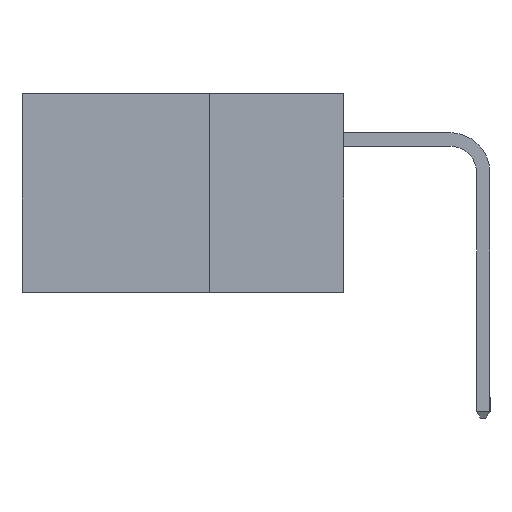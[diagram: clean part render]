
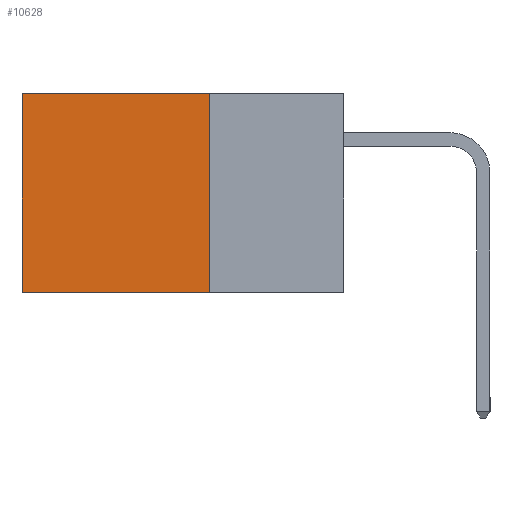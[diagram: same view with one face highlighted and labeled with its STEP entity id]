
A CAD part, left-side view. The second image highlights one B-rep face of the part: STEP entity #10628.
In plain terms, the highlighted planar face has unit normal (-1, 0, 0).
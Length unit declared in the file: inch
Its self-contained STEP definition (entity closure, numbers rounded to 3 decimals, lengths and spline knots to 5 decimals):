
#128 = CARTESIAN_POINT ( 'NONE',  ( 0.2615, 0.6, 0. ) ) ;
#481 = DIRECTION ( 'NONE',  ( 1., 0., 0. ) ) ;
#501 = LINE ( 'NONE', #14628, #19269 ) ;
#578 = EDGE_CURVE ( 'NONE', #7207, #7110, #7001, .T. ) ;
#1462 = CARTESIAN_POINT ( 'NONE',  ( 0.2615, 0.25, -0.37 ) ) ;
#2629 = VECTOR ( 'NONE', #13078, 39.37008 ) ;
#3656 = CARTESIAN_POINT ( 'NONE',  ( 0.2615, 0.6, -0.37 ) ) ;
#3917 = AXIS2_PLACEMENT_3D ( 'NONE', #11691, #481, #13597 ) ;
#5743 = EDGE_CURVE ( 'NONE', #24063, #7207, #501, .T. ) ;
#6727 = LINE ( 'NONE', #1462, #16217 ) ;
#7001 = LINE ( 'NONE', #16262, #2629 ) ;
#7110 = VERTEX_POINT ( 'NONE', #3656 ) ;
#7207 = VERTEX_POINT ( 'NONE', #128 ) ;
#8527 = ORIENTED_EDGE ( 'NONE', *, *, #578, .T. ) ;
#10224 = DIRECTION ( 'NONE',  ( 0., 1., 0. ) ) ;
#10291 = ORIENTED_EDGE ( 'NONE', *, *, #17161, .F. ) ;
#10628 = ADVANCED_FACE ( 'NONE', ( #15994 ), #22792, .F. ) ;
#10825 = CARTESIAN_POINT ( 'NONE',  ( 0.2615, 0.25, -0.37 ) ) ;
#10855 = EDGE_LOOP ( 'NONE', ( #8527, #23419, #10291, #23080 ) ) ;
#11691 = CARTESIAN_POINT ( 'NONE',  ( 0.2615, 0.25, -0.37 ) ) ;
#12715 = DIRECTION ( 'NONE',  ( 0., 0., -1. ) ) ;
#13078 = DIRECTION ( 'NONE',  ( 0., 0., -1. ) ) ;
#13472 = CARTESIAN_POINT ( 'NONE',  ( 0.2615, 0.25, 0. ) ) ;
#13597 = DIRECTION ( 'NONE',  ( 0., 0., -1. ) ) ;
#14628 = CARTESIAN_POINT ( 'NONE',  ( 0.2615, 0.25, 0. ) ) ;
#15573 = CARTESIAN_POINT ( 'NONE',  ( 0.2615, 0.25, -0.37 ) ) ;
#15994 = FACE_OUTER_BOUND ( 'NONE', #10855, .T. ) ;
#16217 = VECTOR ( 'NONE', #16535, 39.37008 ) ;
#16262 = CARTESIAN_POINT ( 'NONE',  ( 0.2615, 0.6, -0.37 ) ) ;
#16535 = DIRECTION ( 'NONE',  ( 0., 1., 0. ) ) ;
#16607 = LINE ( 'NONE', #10825, #20902 ) ;
#17161 = EDGE_CURVE ( 'NONE', #24063, #20299, #16607, .T. ) ;
#19116 = EDGE_CURVE ( 'NONE', #20299, #7110, #6727, .T. ) ;
#19269 = VECTOR ( 'NONE', #10224, 39.37008 ) ;
#20299 = VERTEX_POINT ( 'NONE', #15573 ) ;
#20902 = VECTOR ( 'NONE', #12715, 39.37008 ) ;
#22792 = PLANE ( 'NONE',  #3917 ) ;
#23080 = ORIENTED_EDGE ( 'NONE', *, *, #5743, .T. ) ;
#23419 = ORIENTED_EDGE ( 'NONE', *, *, #19116, .F. ) ;
#24063 = VERTEX_POINT ( 'NONE', #13472 ) ;
